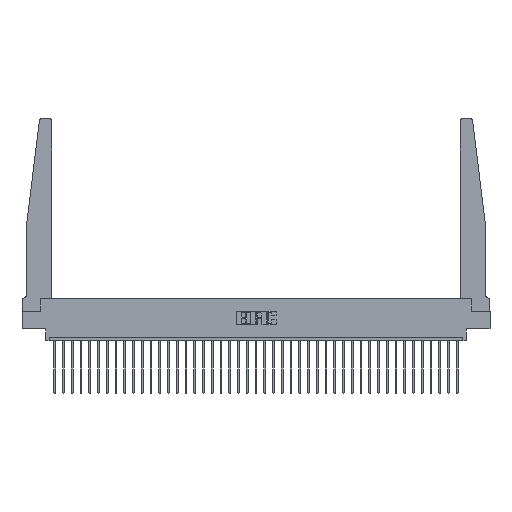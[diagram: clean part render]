
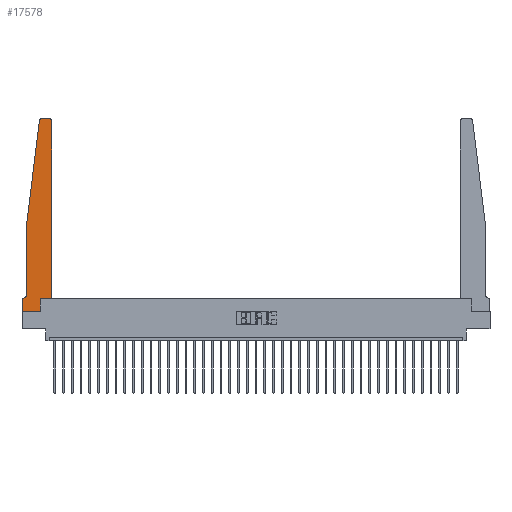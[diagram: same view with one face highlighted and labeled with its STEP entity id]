
A CAD part, top view. The second image highlights one B-rep face of the part: STEP entity #17578.
In plain terms, the highlighted planar face has unit normal (0, 0, 1).
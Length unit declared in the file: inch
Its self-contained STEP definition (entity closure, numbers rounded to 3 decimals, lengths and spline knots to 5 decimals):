
#470 = LINE ( 'NONE', #31969, #15211 ) ;
#586 = CARTESIAN_POINT ( 'NONE',  ( 0.425, 0.18, 0.37 ) ) ;
#620 = ORIENTED_EDGE ( 'NONE', *, *, #14151, .T. ) ;
#1089 = ORIENTED_EDGE ( 'NONE', *, *, #12518, .T. ) ;
#1216 = VERTEX_POINT ( 'NONE', #2539 ) ;
#1244 = EDGE_CURVE ( 'NONE', #1561, #21660, #470, .T. ) ;
#1561 = VERTEX_POINT ( 'NONE', #10195 ) ;
#1714 = VERTEX_POINT ( 'NONE', #586 ) ;
#2539 = CARTESIAN_POINT ( 'NONE',  ( 0., 0., 0.37 ) ) ;
#2611 = CIRCLE ( 'NONE', #33220, 0.05 ) ;
#2935 = DIRECTION ( 'NONE',  ( -0.122, -0.992, 0. ) ) ;
#3382 = VERTEX_POINT ( 'NONE', #10161 ) ;
#4398 = CARTESIAN_POINT ( 'NONE',  ( 0.395, 2.72, 0.37 ) ) ;
#5131 = CARTESIAN_POINT ( 'NONE',  ( 0.27653, 2.75, 0.37 ) ) ;
#6288 = CARTESIAN_POINT ( 'NONE',  ( 0.425, 2.72, 0.37 ) ) ;
#6424 = DIRECTION ( 'NONE',  ( -1., 0., 0. ) ) ;
#6942 = ORIENTED_EDGE ( 'NONE', *, *, #1244, .T. ) ;
#7183 = ORIENTED_EDGE ( 'NONE', *, *, #10277, .T. ) ;
#7733 = LINE ( 'NONE', #28781, #33727 ) ;
#8227 = PLANE ( 'NONE',  #27861 ) ;
#8921 = DIRECTION ( 'NONE',  ( 0., -1., 0. ) ) ;
#9203 = ORIENTED_EDGE ( 'NONE', *, *, #25612, .T. ) ;
#9516 = DIRECTION ( 'NONE',  ( 0., 0., 1. ) ) ;
#9588 = ORIENTED_EDGE ( 'NONE', *, *, #28508, .T. ) ;
#9724 = DIRECTION ( 'NONE',  ( 1., 0., 0. ) ) ;
#9736 = VECTOR ( 'NONE', #2935, 39.37008 ) ;
#10161 = CARTESIAN_POINT ( 'NONE',  ( 0.395, 2.75, 0.37 ) ) ;
#10195 = CARTESIAN_POINT ( 'NONE',  ( 0.015, 0.1875, 0.37 ) ) ;
#10277 = EDGE_CURVE ( 'NONE', #30532, #30762, #14497, .T. ) ;
#10310 = LINE ( 'NONE', #21399, #9736 ) ;
#10725 = LINE ( 'NONE', #33667, #23767 ) ;
#11904 = LINE ( 'NONE', #14480, #28683 ) ;
#11949 = CARTESIAN_POINT ( 'NONE',  ( 0.24675, 2.72367, 0.37 ) ) ;
#12100 = AXIS2_PLACEMENT_3D ( 'NONE', #4398, #9516, #19942 ) ;
#12518 = EDGE_CURVE ( 'NONE', #1216, #29260, #7733, .T. ) ;
#12944 = ORIENTED_EDGE ( 'NONE', *, *, #33299, .T. ) ;
#13137 = VERTEX_POINT ( 'NONE', #6288 ) ;
#14151 = EDGE_CURVE ( 'NONE', #30762, #26062, #10310, .T. ) ;
#14480 = CARTESIAN_POINT ( 'NONE',  ( 0.2605, 0.18, 0.37 ) ) ;
#14497 = CIRCLE ( 'NONE', #21045, 0.03 ) ;
#14685 = EDGE_CURVE ( 'NONE', #1714, #13137, #32604, .T. ) ;
#15211 = VECTOR ( 'NONE', #16697, 39.37008 ) ;
#16155 = CARTESIAN_POINT ( 'NONE',  ( 0.27653, 2.72, 0.37 ) ) ;
#16468 = DIRECTION ( 'NONE',  ( -1., 0., 0. ) ) ;
#16697 = DIRECTION ( 'NONE',  ( -1., 0., 0. ) ) ;
#16974 = CARTESIAN_POINT ( 'NONE',  ( 0.065, 1.25, 0.37 ) ) ;
#17578 = ADVANCED_FACE ( 'NONE', ( #31684 ), #8227, .T. ) ;
#18383 = DIRECTION ( 'NONE',  ( 1., 0., 0. ) ) ;
#19112 = VERTEX_POINT ( 'NONE', #31311 ) ;
#19266 = CARTESIAN_POINT ( 'NONE',  ( 0.25, 2.75, 0.37 ) ) ;
#19872 = LINE ( 'NONE', #33248, #29798 ) ;
#19942 = DIRECTION ( 'NONE',  ( 1., 0., 0. ) ) ;
#20076 = ORIENTED_EDGE ( 'NONE', *, *, #14685, .T. ) ;
#20558 = EDGE_LOOP ( 'NONE', ( #33761, #7183, #620, #24471, #9588, #6942, #12944, #1089, #9203, #26872, #20076, #33507 ) ) ;
#20792 = EDGE_CURVE ( 'NONE', #13137, #3382, #21382, .T. ) ;
#21045 = AXIS2_PLACEMENT_3D ( 'NONE', #16155, #29507, #18383 ) ;
#21382 = CIRCLE ( 'NONE', #12100, 0.03 ) ;
#21399 = CARTESIAN_POINT ( 'NONE',  ( 0.065, 1.25, 0.37 ) ) ;
#21651 = LINE ( 'NONE', #19266, #23428 ) ;
#21660 = VERTEX_POINT ( 'NONE', #22604 ) ;
#21914 = LINE ( 'NONE', #22074, #25649 ) ;
#22074 = CARTESIAN_POINT ( 'NONE',  ( 0., 0., 0.37 ) ) ;
#22539 = CARTESIAN_POINT ( 'NONE',  ( 0.065, 0.2375, 0.37 ) ) ;
#22604 = CARTESIAN_POINT ( 'NONE',  ( 0., 0.1875, 0.37 ) ) ;
#23428 = VECTOR ( 'NONE', #6424, 39.37008 ) ;
#23767 = VECTOR ( 'NONE', #26450, 39.37008 ) ;
#24034 = EDGE_CURVE ( 'NONE', #19112, #1714, #10725, .T. ) ;
#24329 = CARTESIAN_POINT ( 'NONE',  ( 0.015, 0.2375, 0.37 ) ) ;
#24471 = ORIENTED_EDGE ( 'NONE', *, *, #26055, .T. ) ;
#25013 = DIRECTION ( 'NONE',  ( 0., -1., 0. ) ) ;
#25517 = VECTOR ( 'NONE', #32783, 39.37008 ) ;
#25612 = EDGE_CURVE ( 'NONE', #29260, #19112, #11904, .T. ) ;
#25649 = VECTOR ( 'NONE', #8921, 39.37008 ) ;
#26055 = EDGE_CURVE ( 'NONE', #26062, #32207, #19872, .T. ) ;
#26062 = VERTEX_POINT ( 'NONE', #16974 ) ;
#26450 = DIRECTION ( 'NONE',  ( 1., 0., 0. ) ) ;
#26872 = ORIENTED_EDGE ( 'NONE', *, *, #24034, .T. ) ;
#27606 = DIRECTION ( 'NONE',  ( 1., 0., 0. ) ) ;
#27861 = AXIS2_PLACEMENT_3D ( 'NONE', #29116, #29942, #9724 ) ;
#28508 = EDGE_CURVE ( 'NONE', #32207, #1561, #2611, .T. ) ;
#28683 = VECTOR ( 'NONE', #33462, 39.37008 ) ;
#28781 = CARTESIAN_POINT ( 'NONE',  ( 0., 0., 0.37 ) ) ;
#29116 = CARTESIAN_POINT ( 'NONE',  ( 0., 0.1875, 0.37 ) ) ;
#29260 = VERTEX_POINT ( 'NONE', #33840 ) ;
#29507 = DIRECTION ( 'NONE',  ( 0., 0., 1. ) ) ;
#29798 = VECTOR ( 'NONE', #25013, 39.37008 ) ;
#29942 = DIRECTION ( 'NONE',  ( 0., 0., 1. ) ) ;
#30532 = VERTEX_POINT ( 'NONE', #5131 ) ;
#30762 = VERTEX_POINT ( 'NONE', #11949 ) ;
#31246 = EDGE_CURVE ( 'NONE', #3382, #30532, #21651, .T. ) ;
#31311 = CARTESIAN_POINT ( 'NONE',  ( 0.2605, 0.18, 0.37 ) ) ;
#31684 = FACE_OUTER_BOUND ( 'NONE', #20558, .T. ) ;
#31892 = DIRECTION ( 'NONE',  ( 0., 0., -1. ) ) ;
#31969 = CARTESIAN_POINT ( 'NONE',  ( 0.065, 0.1875, 0.37 ) ) ;
#32207 = VERTEX_POINT ( 'NONE', #22539 ) ;
#32444 = CARTESIAN_POINT ( 'NONE',  ( 0.425, 0.18, 0.37 ) ) ;
#32604 = LINE ( 'NONE', #32444, #25517 ) ;
#32783 = DIRECTION ( 'NONE',  ( 0., 1., 0. ) ) ;
#33220 = AXIS2_PLACEMENT_3D ( 'NONE', #24329, #31892, #16468 ) ;
#33248 = CARTESIAN_POINT ( 'NONE',  ( 0.065, 1.25, 0.37 ) ) ;
#33299 = EDGE_CURVE ( 'NONE', #21660, #1216, #21914, .T. ) ;
#33462 = DIRECTION ( 'NONE',  ( 0., 1., 0. ) ) ;
#33507 = ORIENTED_EDGE ( 'NONE', *, *, #20792, .T. ) ;
#33667 = CARTESIAN_POINT ( 'NONE',  ( 0.425, 0.18, 0.37 ) ) ;
#33727 = VECTOR ( 'NONE', #27606, 39.37008 ) ;
#33761 = ORIENTED_EDGE ( 'NONE', *, *, #31246, .T. ) ;
#33840 = CARTESIAN_POINT ( 'NONE',  ( 0.2605, 0., 0.37 ) ) ;
